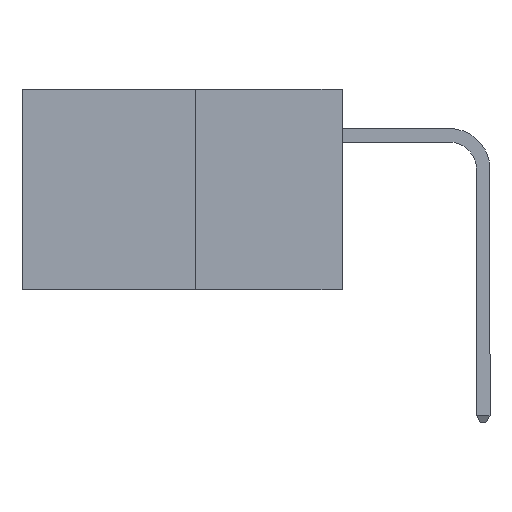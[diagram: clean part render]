
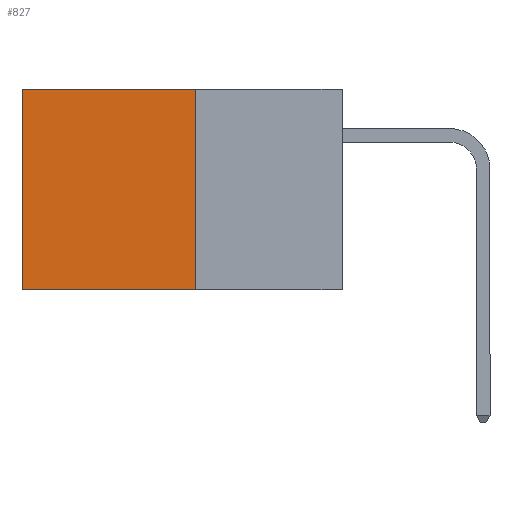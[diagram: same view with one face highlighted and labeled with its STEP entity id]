
A CAD part, left-side view. The second image highlights one B-rep face of the part: STEP entity #827.
In plain terms, the highlighted planar face has unit normal (-1, 0, 0).
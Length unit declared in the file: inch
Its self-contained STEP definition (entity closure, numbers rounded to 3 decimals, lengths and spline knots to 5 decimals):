
#123 = CARTESIAN_POINT ( 'NONE',  ( 0.277, 0.59, -0.37 ) ) ;
#217 = DIRECTION ( 'NONE',  ( 1., 0., 0. ) ) ;
#310 = VERTEX_POINT ( 'NONE', #2793 ) ;
#662 = VERTEX_POINT ( 'NONE', #7632 ) ;
#804 = CARTESIAN_POINT ( 'NONE',  ( 0.277, 0.27, -0.37 ) ) ;
#827 = ADVANCED_FACE ( 'NONE', ( #3652 ), #6841, .F. ) ;
#1386 = DIRECTION ( 'NONE',  ( 0., 0., -1. ) ) ;
#1623 = CARTESIAN_POINT ( 'NONE',  ( 0.277, 0.27, -0.37 ) ) ;
#2165 = LINE ( 'NONE', #123, #6913 ) ;
#2624 = VECTOR ( 'NONE', #5674, 39.37008 ) ;
#2650 = ORIENTED_EDGE ( 'NONE', *, *, #8066, .F. ) ;
#2793 = CARTESIAN_POINT ( 'NONE',  ( 0.277, 0.59, 0. ) ) ;
#2980 = DIRECTION ( 'NONE',  ( 0., 0., -1. ) ) ;
#3129 = VECTOR ( 'NONE', #4342, 39.37008 ) ;
#3305 = ORIENTED_EDGE ( 'NONE', *, *, #4047, .T. ) ;
#3499 = EDGE_CURVE ( 'NONE', #662, #310, #4777, .T. ) ;
#3639 = ORIENTED_EDGE ( 'NONE', *, *, #3499, .T. ) ;
#3652 = FACE_OUTER_BOUND ( 'NONE', #7901, .T. ) ;
#4047 = EDGE_CURVE ( 'NONE', #310, #4952, #2165, .T. ) ;
#4342 = DIRECTION ( 'NONE',  ( 0., 1., 0. ) ) ;
#4346 = ORIENTED_EDGE ( 'NONE', *, *, #7983, .F. ) ;
#4379 = CARTESIAN_POINT ( 'NONE',  ( 0.277, 0.27, 0. ) ) ;
#4502 = LINE ( 'NONE', #4925, #2624 ) ;
#4654 = CARTESIAN_POINT ( 'NONE',  ( 0.277, 0.59, -0.37 ) ) ;
#4777 = LINE ( 'NONE', #4379, #3129 ) ;
#4925 = CARTESIAN_POINT ( 'NONE',  ( 0.277, 0.27, -0.37 ) ) ;
#4952 = VERTEX_POINT ( 'NONE', #4654 ) ;
#5674 = DIRECTION ( 'NONE',  ( 0., 1., 0. ) ) ;
#6289 = VECTOR ( 'NONE', #1386, 39.37008 ) ;
#6422 = CARTESIAN_POINT ( 'NONE',  ( 0.277, 0.27, -0.37 ) ) ;
#6524 = AXIS2_PLACEMENT_3D ( 'NONE', #804, #217, #2980 ) ;
#6841 = PLANE ( 'NONE',  #6524 ) ;
#6913 = VECTOR ( 'NONE', #7367, 39.37008 ) ;
#7367 = DIRECTION ( 'NONE',  ( 0., 0., -1. ) ) ;
#7632 = CARTESIAN_POINT ( 'NONE',  ( 0.277, 0.27, 0. ) ) ;
#7841 = LINE ( 'NONE', #1623, #6289 ) ;
#7901 = EDGE_LOOP ( 'NONE', ( #3305, #2650, #4346, #3639 ) ) ;
#7983 = EDGE_CURVE ( 'NONE', #662, #8261, #7841, .T. ) ;
#8066 = EDGE_CURVE ( 'NONE', #8261, #4952, #4502, .T. ) ;
#8261 = VERTEX_POINT ( 'NONE', #6422 ) ;
